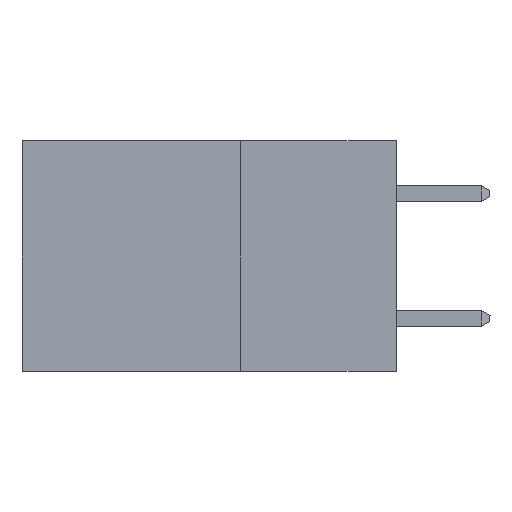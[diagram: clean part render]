
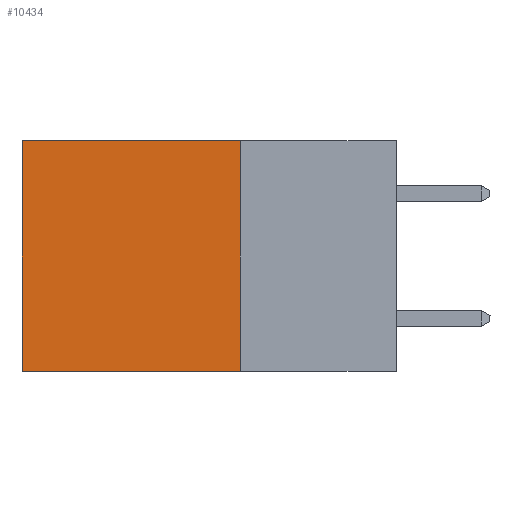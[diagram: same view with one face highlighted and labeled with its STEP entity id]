
A CAD part, left-side view. The second image highlights one B-rep face of the part: STEP entity #10434.
In plain terms, the highlighted planar face has unit normal (-1, 0, 0).
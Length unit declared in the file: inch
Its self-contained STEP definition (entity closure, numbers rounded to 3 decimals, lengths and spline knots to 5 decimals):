
#707 = PLANE ( 'NONE',  #6946 ) ;
#924 = CARTESIAN_POINT ( 'NONE',  ( 0.2615, 0.25, 0. ) ) ;
#1031 = EDGE_CURVE ( 'NONE', #8496, #14573, #4482, .T. ) ;
#1917 = DIRECTION ( 'NONE',  ( 0., 0., -1. ) ) ;
#2612 = DIRECTION ( 'NONE',  ( 0., 0., -1. ) ) ;
#2780 = CARTESIAN_POINT ( 'NONE',  ( 0.2615, 0.25, -0.37 ) ) ;
#2816 = VECTOR ( 'NONE', #2612, 39.37008 ) ;
#3382 = VECTOR ( 'NONE', #9987, 39.37008 ) ;
#3553 = EDGE_CURVE ( 'NONE', #14754, #8496, #6111, .T. ) ;
#4482 = LINE ( 'NONE', #10587, #10856 ) ;
#4658 = EDGE_LOOP ( 'NONE', ( #11895, #5585, #8781, #9784 ) ) ;
#4943 = VECTOR ( 'NONE', #14094, 39.37008 ) ;
#5124 = EDGE_CURVE ( 'NONE', #14777, #14573, #11276, .T. ) ;
#5585 = ORIENTED_EDGE ( 'NONE', *, *, #1031, .F. ) ;
#6111 = LINE ( 'NONE', #2780, #2816 ) ;
#6633 = LINE ( 'NONE', #10153, #3382 ) ;
#6946 = AXIS2_PLACEMENT_3D ( 'NONE', #13943, #9249, #1917 ) ;
#7095 = CARTESIAN_POINT ( 'NONE',  ( 0.2615, 0.6, 0. ) ) ;
#7580 = DIRECTION ( 'NONE',  ( 0., 1., 0. ) ) ;
#8496 = VERTEX_POINT ( 'NONE', #10068 ) ;
#8497 = EDGE_CURVE ( 'NONE', #14754, #14777, #6633, .T. ) ;
#8781 = ORIENTED_EDGE ( 'NONE', *, *, #3553, .F. ) ;
#9249 = DIRECTION ( 'NONE',  ( 1., 0., 0. ) ) ;
#9784 = ORIENTED_EDGE ( 'NONE', *, *, #8497, .T. ) ;
#9987 = DIRECTION ( 'NONE',  ( 0., 1., 0. ) ) ;
#10068 = CARTESIAN_POINT ( 'NONE',  ( 0.2615, 0.25, -0.37 ) ) ;
#10153 = CARTESIAN_POINT ( 'NONE',  ( 0.2615, 0.25, 0. ) ) ;
#10335 = CARTESIAN_POINT ( 'NONE',  ( 0.2615, 0.6, -0.37 ) ) ;
#10434 = ADVANCED_FACE ( 'NONE', ( #11970 ), #707, .F. ) ;
#10587 = CARTESIAN_POINT ( 'NONE',  ( 0.2615, 0.25, -0.37 ) ) ;
#10856 = VECTOR ( 'NONE', #7580, 39.37008 ) ;
#11276 = LINE ( 'NONE', #13999, #4943 ) ;
#11895 = ORIENTED_EDGE ( 'NONE', *, *, #5124, .T. ) ;
#11970 = FACE_OUTER_BOUND ( 'NONE', #4658, .T. ) ;
#13943 = CARTESIAN_POINT ( 'NONE',  ( 0.2615, 0.25, -0.37 ) ) ;
#13999 = CARTESIAN_POINT ( 'NONE',  ( 0.2615, 0.6, -0.37 ) ) ;
#14094 = DIRECTION ( 'NONE',  ( 0., 0., -1. ) ) ;
#14573 = VERTEX_POINT ( 'NONE', #10335 ) ;
#14754 = VERTEX_POINT ( 'NONE', #924 ) ;
#14777 = VERTEX_POINT ( 'NONE', #7095 ) ;
